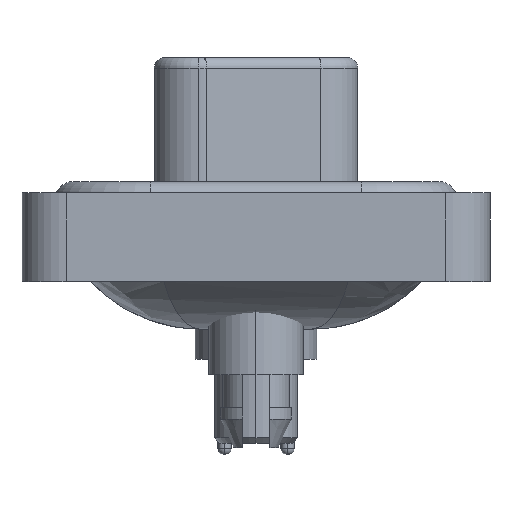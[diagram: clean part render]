
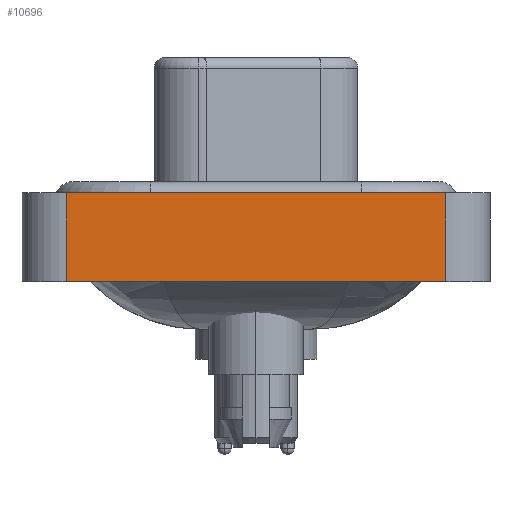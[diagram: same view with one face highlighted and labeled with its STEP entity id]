
A CAD part, left-side view. The second image highlights one B-rep face of the part: STEP entity #10696.
In plain terms, the highlighted planar face has unit normal (-1, 0, 0).
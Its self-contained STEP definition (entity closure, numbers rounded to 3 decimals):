
#550 = ORIENTED_EDGE ( 'NONE', *, *, #5738, .T. ) ;
#809 = LINE ( 'NONE', #9017, #19218 ) ;
#941 = DIRECTION ( 'NONE',  ( 0., 0., 1. ) ) ;
#2876 = CARTESIAN_POINT ( 'NONE',  ( -7.35, 8.55, -3.6 ) ) ;
#3458 = LINE ( 'NONE', #3979, #20589 ) ;
#3607 = VERTEX_POINT ( 'NONE', #18381 ) ;
#3979 = CARTESIAN_POINT ( 'NONE',  ( -7.35, -8.55, -3.6 ) ) ;
#5461 = VECTOR ( 'NONE', #14473, 1000. ) ;
#5738 = EDGE_CURVE ( 'NONE', #18535, #15469, #15470, .T. ) ;
#7188 = DIRECTION ( 'NONE',  ( -1., 0., 0. ) ) ;
#8944 = PLANE ( 'NONE',  #19877 ) ;
#9017 = CARTESIAN_POINT ( 'NONE',  ( -7.35, -8.55, 0.4 ) ) ;
#9697 = EDGE_CURVE ( 'NONE', #3607, #18535, #3458, .T. ) ;
#10672 = CARTESIAN_POINT ( 'NONE',  ( -7.35, -8.55, -3.6 ) ) ;
#10696 = ADVANCED_FACE ( 'NONE', ( #19209 ), #8944, .T. ) ;
#12321 = DIRECTION ( 'NONE',  ( 0., 0., 1. ) ) ;
#13169 = CARTESIAN_POINT ( 'NONE',  ( -7.35, -8.55, 0.4 ) ) ;
#13511 = VECTOR ( 'NONE', #12321, 1000. ) ;
#14059 = DIRECTION ( 'NONE',  ( 0., -1., 0. ) ) ;
#14473 = DIRECTION ( 'NONE',  ( 0., 0., 1. ) ) ;
#15469 = VERTEX_POINT ( 'NONE', #13169 ) ;
#15470 = LINE ( 'NONE', #10672, #13511 ) ;
#15675 = ORIENTED_EDGE ( 'NONE', *, *, #9697, .T. ) ;
#15722 = CARTESIAN_POINT ( 'NONE',  ( -7.35, -8.55, -3.6 ) ) ;
#15779 = ORIENTED_EDGE ( 'NONE', *, *, #18155, .F. ) ;
#16216 = LINE ( 'NONE', #2876, #5461 ) ;
#17096 = ORIENTED_EDGE ( 'NONE', *, *, #20640, .F. ) ;
#17313 = DIRECTION ( 'NONE',  ( 0., -1., 0. ) ) ;
#17590 = CARTESIAN_POINT ( 'NONE',  ( -7.35, 8.55, 0.4 ) ) ;
#17824 = CARTESIAN_POINT ( 'NONE',  ( -7.35, -8.55, -3.6 ) ) ;
#18155 = EDGE_CURVE ( 'NONE', #3607, #21031, #16216, .T. ) ;
#18381 = CARTESIAN_POINT ( 'NONE',  ( -7.35, 8.55, -3.6 ) ) ;
#18535 = VERTEX_POINT ( 'NONE', #17824 ) ;
#19209 = FACE_OUTER_BOUND ( 'NONE', #19785, .T. ) ;
#19218 = VECTOR ( 'NONE', #14059, 1000. ) ;
#19785 = EDGE_LOOP ( 'NONE', ( #550, #17096, #15779, #15675 ) ) ;
#19877 = AXIS2_PLACEMENT_3D ( 'NONE', #15722, #7188, #941 ) ;
#20589 = VECTOR ( 'NONE', #17313, 1000. ) ;
#20640 = EDGE_CURVE ( 'NONE', #21031, #15469, #809, .T. ) ;
#21031 = VERTEX_POINT ( 'NONE', #17590 ) ;
